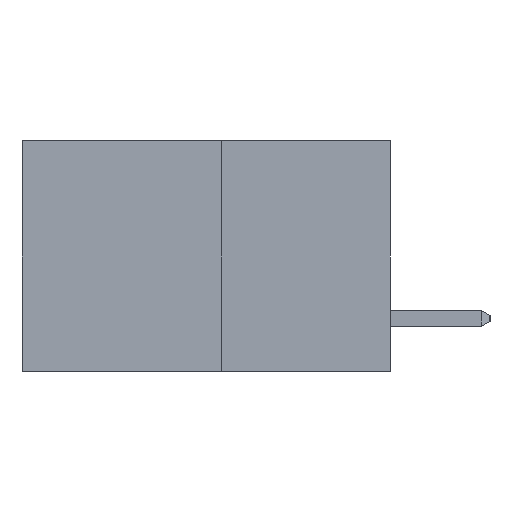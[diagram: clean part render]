
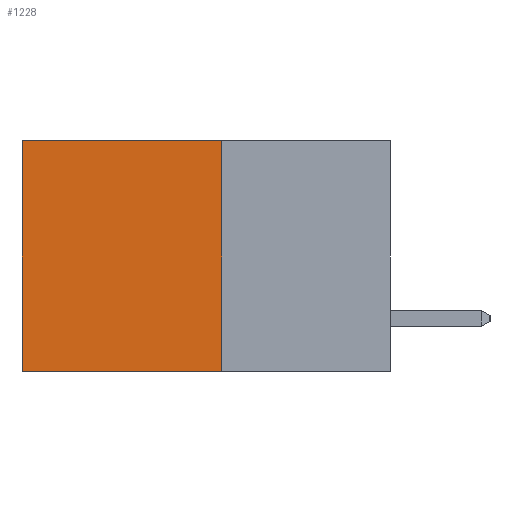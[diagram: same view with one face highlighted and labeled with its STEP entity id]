
A CAD part, left-side view. The second image highlights one B-rep face of the part: STEP entity #1228.
In plain terms, the highlighted planar face has unit normal (-1, 0, 0).
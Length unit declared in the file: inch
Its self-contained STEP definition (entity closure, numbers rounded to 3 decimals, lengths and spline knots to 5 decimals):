
#556 = CARTESIAN_POINT ( 'NONE',  ( 0.277, 0.27, 0. ) ) ;
#1228 = ADVANCED_FACE ( 'NONE', ( #20533 ), #18407, .F. ) ;
#1429 = LINE ( 'NONE', #16559, #2514 ) ;
#2295 = DIRECTION ( 'NONE',  ( 0., 1., 0. ) ) ;
#2337 = DIRECTION ( 'NONE',  ( 0., 0., -1. ) ) ;
#2514 = VECTOR ( 'NONE', #16625, 39.37008 ) ;
#3999 = EDGE_CURVE ( 'NONE', #5476, #16388, #13388, .T. ) ;
#4279 = ORIENTED_EDGE ( 'NONE', *, *, #11683, .T. ) ;
#4620 = EDGE_CURVE ( 'NONE', #14599, #18733, #5457, .T. ) ;
#5421 = CARTESIAN_POINT ( 'NONE',  ( 0.277, 0.59, -0.37 ) ) ;
#5457 = LINE ( 'NONE', #11412, #14443 ) ;
#5476 = VERTEX_POINT ( 'NONE', #7381 ) ;
#7381 = CARTESIAN_POINT ( 'NONE',  ( 0.277, 0.59, 0. ) ) ;
#10140 = EDGE_CURVE ( 'NONE', #18733, #16388, #1429, .T. ) ;
#10265 = CARTESIAN_POINT ( 'NONE',  ( 0.277, 0.59, -0.37 ) ) ;
#10314 = CARTESIAN_POINT ( 'NONE',  ( 0.277, 0.27, -0.37 ) ) ;
#11412 = CARTESIAN_POINT ( 'NONE',  ( 0.277, 0.27, -0.37 ) ) ;
#11683 = EDGE_CURVE ( 'NONE', #14599, #5476, #12530, .T. ) ;
#12059 = DIRECTION ( 'NONE',  ( 0., 0., -1. ) ) ;
#12530 = LINE ( 'NONE', #556, #20849 ) ;
#12678 = CARTESIAN_POINT ( 'NONE',  ( 0.277, 0.27, 0. ) ) ;
#12759 = EDGE_LOOP ( 'NONE', ( #18518, #20298, #20208, #4279 ) ) ;
#13388 = LINE ( 'NONE', #5421, #21698 ) ;
#14443 = VECTOR ( 'NONE', #12059, 39.37008 ) ;
#14599 = VERTEX_POINT ( 'NONE', #12678 ) ;
#15683 = AXIS2_PLACEMENT_3D ( 'NONE', #20547, #20390, #20568 ) ;
#16388 = VERTEX_POINT ( 'NONE', #10265 ) ;
#16559 = CARTESIAN_POINT ( 'NONE',  ( 0.277, 0.27, -0.37 ) ) ;
#16625 = DIRECTION ( 'NONE',  ( 0., 1., 0. ) ) ;
#18407 = PLANE ( 'NONE',  #15683 ) ;
#18518 = ORIENTED_EDGE ( 'NONE', *, *, #3999, .T. ) ;
#18733 = VERTEX_POINT ( 'NONE', #10314 ) ;
#20208 = ORIENTED_EDGE ( 'NONE', *, *, #4620, .F. ) ;
#20298 = ORIENTED_EDGE ( 'NONE', *, *, #10140, .F. ) ;
#20390 = DIRECTION ( 'NONE',  ( 1., 0., 0. ) ) ;
#20533 = FACE_OUTER_BOUND ( 'NONE', #12759, .T. ) ;
#20547 = CARTESIAN_POINT ( 'NONE',  ( 0.277, 0.27, -0.37 ) ) ;
#20568 = DIRECTION ( 'NONE',  ( 0., 0., -1. ) ) ;
#20849 = VECTOR ( 'NONE', #2295, 39.37008 ) ;
#21698 = VECTOR ( 'NONE', #2337, 39.37008 ) ;
